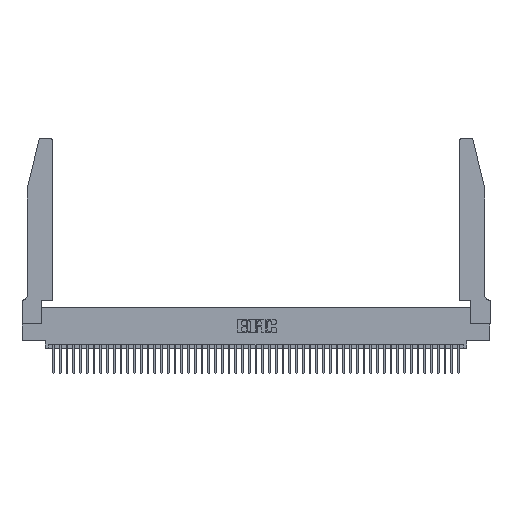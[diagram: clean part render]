
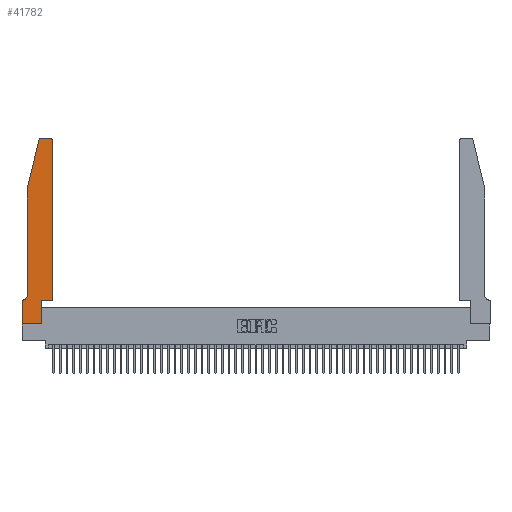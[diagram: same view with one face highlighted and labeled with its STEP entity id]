
A CAD part, top view. The second image highlights one B-rep face of the part: STEP entity #41782.
In plain terms, the highlighted planar face has unit normal (0, 0, 1).
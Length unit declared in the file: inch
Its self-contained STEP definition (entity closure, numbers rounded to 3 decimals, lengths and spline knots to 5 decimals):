
#335 = DIRECTION ( 'NONE',  ( 0., 0., 1. ) ) ;
#446 = VECTOR ( 'NONE', #50168, 39.37008 ) ;
#888 = ORIENTED_EDGE ( 'NONE', *, *, #5097, .T. ) ;
#3305 = ORIENTED_EDGE ( 'NONE', *, *, #12904, .T. ) ;
#3406 = EDGE_CURVE ( 'NONE', #11469, #32668, #41347, .T. ) ;
#3978 = VERTEX_POINT ( 'NONE', #6735 ) ;
#4355 = LINE ( 'NONE', #41577, #32899 ) ;
#4469 = DIRECTION ( 'NONE',  ( 0., 0., -1. ) ) ;
#5052 = VECTOR ( 'NONE', #42240, 39.37008 ) ;
#5097 = EDGE_CURVE ( 'NONE', #18973, #18707, #19340, .T. ) ;
#5309 = DIRECTION ( 'NONE',  ( 0., 0., 1. ) ) ;
#5389 = LINE ( 'NONE', #21109, #25408 ) ;
#5533 = EDGE_CURVE ( 'NONE', #21859, #3978, #30871, .T. ) ;
#6735 = CARTESIAN_POINT ( 'NONE',  ( 0.4205, 2.75, 0.37 ) ) ;
#6910 = EDGE_CURVE ( 'NONE', #35512, #21859, #24054, .T. ) ;
#7322 = CARTESIAN_POINT ( 'NONE',  ( 0., 0., 0.37 ) ) ;
#8686 = AXIS2_PLACEMENT_3D ( 'NONE', #47354, #4469, #46852 ) ;
#10086 = EDGE_CURVE ( 'NONE', #29222, #35360, #40199, .T. ) ;
#10791 = CARTESIAN_POINT ( 'NONE',  ( 0.284, 2.75, 0.37 ) ) ;
#11469 = VERTEX_POINT ( 'NONE', #32171 ) ;
#11515 = CARTESIAN_POINT ( 'NONE',  ( 0.4505, 0.35, 0.37 ) ) ;
#12031 = CARTESIAN_POINT ( 'NONE',  ( 0.0755, 0.42, 0.37 ) ) ;
#12190 = CARTESIAN_POINT ( 'NONE',  ( 0.4505, 0.35, 0.37 ) ) ;
#12241 = CARTESIAN_POINT ( 'NONE',  ( 0.4505, 2.72, 0.37 ) ) ;
#12771 = VERTEX_POINT ( 'NONE', #32557 ) ;
#12904 = EDGE_CURVE ( 'NONE', #12771, #30548, #36327, .T. ) ;
#13522 = ORIENTED_EDGE ( 'NONE', *, *, #5533, .T. ) ;
#13536 = LINE ( 'NONE', #14975, #5052 ) ;
#13744 = VECTOR ( 'NONE', #50152, 39.37008 ) ;
#14975 = CARTESIAN_POINT ( 'NONE',  ( 0., 0., 0.37 ) ) ;
#16902 = DIRECTION ( 'NONE',  ( -0.239, -0.971, 0. ) ) ;
#17101 = DIRECTION ( 'NONE',  ( 0., 0., 1. ) ) ;
#17632 = CARTESIAN_POINT ( 'NONE',  ( 0.0755, 0.35, 0.37 ) ) ;
#18300 = ORIENTED_EDGE ( 'NONE', *, *, #29559, .T. ) ;
#18707 = VERTEX_POINT ( 'NONE', #44211 ) ;
#18973 = VERTEX_POINT ( 'NONE', #10791 ) ;
#19340 = CIRCLE ( 'NONE', #34306, 0.03 ) ;
#19495 = EDGE_CURVE ( 'NONE', #35360, #35512, #4355, .T. ) ;
#20684 = EDGE_LOOP ( 'NONE', ( #49990, #888, #25236, #41592, #18300, #3305, #41194, #24878, #39655, #31761, #39203, #13522 ) ) ;
#20696 = CARTESIAN_POINT ( 'NONE',  ( 0., 0., 0.37 ) ) ;
#21109 = CARTESIAN_POINT ( 'NONE',  ( 0.0755, 2., 0.37 ) ) ;
#21523 = DIRECTION ( 'NONE',  ( -1., 0., 0. ) ) ;
#21859 = VERTEX_POINT ( 'NONE', #12241 ) ;
#21994 = CIRCLE ( 'NONE', #8686, 0.07 ) ;
#23254 = CARTESIAN_POINT ( 'NONE',  ( 0.284, 2.72, 0.37 ) ) ;
#24054 = LINE ( 'NONE', #12190, #13744 ) ;
#24582 = AXIS2_PLACEMENT_3D ( 'NONE', #40627, #17101, #29290 ) ;
#24878 = ORIENTED_EDGE ( 'NONE', *, *, #46065, .T. ) ;
#25236 = ORIENTED_EDGE ( 'NONE', *, *, #45693, .T. ) ;
#25249 = EDGE_CURVE ( 'NONE', #3978, #18973, #26533, .T. ) ;
#25408 = VECTOR ( 'NONE', #16902, 39.37008 ) ;
#26160 = DIRECTION ( 'NONE',  ( 1., 0., 0. ) ) ;
#26533 = LINE ( 'NONE', #34922, #446 ) ;
#26850 = VECTOR ( 'NONE', #31368, 39.37008 ) ;
#27152 = CARTESIAN_POINT ( 'NONE',  ( 0.2865, 0.35, 0.37 ) ) ;
#28473 = PLANE ( 'NONE',  #40858 ) ;
#29057 = LINE ( 'NONE', #7322, #45968 ) ;
#29222 = VERTEX_POINT ( 'NONE', #31750 ) ;
#29290 = DIRECTION ( 'NONE',  ( 1., 0., 0. ) ) ;
#29559 = EDGE_CURVE ( 'NONE', #32668, #12771, #21994, .T. ) ;
#30073 = DIRECTION ( 'NONE',  ( 1., 0., 0. ) ) ;
#30548 = VERTEX_POINT ( 'NONE', #45387 ) ;
#30871 = CIRCLE ( 'NONE', #24582, 0.03 ) ;
#31368 = DIRECTION ( 'NONE',  ( 0., 1., 0. ) ) ;
#31750 = CARTESIAN_POINT ( 'NONE',  ( 0.2865, 0., 0.37 ) ) ;
#31761 = ORIENTED_EDGE ( 'NONE', *, *, #19495, .T. ) ;
#32171 = CARTESIAN_POINT ( 'NONE',  ( 0.0755, 2., 0.37 ) ) ;
#32557 = CARTESIAN_POINT ( 'NONE',  ( 0.0055, 0.35, 0.37 ) ) ;
#32668 = VERTEX_POINT ( 'NONE', #12031 ) ;
#32899 = VECTOR ( 'NONE', #30073, 39.37008 ) ;
#33921 = VECTOR ( 'NONE', #21523, 39.37008 ) ;
#34306 = AXIS2_PLACEMENT_3D ( 'NONE', #23254, #335, #43058 ) ;
#34922 = CARTESIAN_POINT ( 'NONE',  ( 0.2605, 2.75, 0.37 ) ) ;
#35360 = VERTEX_POINT ( 'NONE', #44422 ) ;
#35512 = VERTEX_POINT ( 'NONE', #11515 ) ;
#36327 = LINE ( 'NONE', #17632, #33921 ) ;
#36858 = EDGE_CURVE ( 'NONE', #30548, #49402, #13536, .T. ) ;
#37831 = CARTESIAN_POINT ( 'NONE',  ( 0.0755, 2., 0.37 ) ) ;
#38915 = VECTOR ( 'NONE', #50025, 39.37008 ) ;
#39203 = ORIENTED_EDGE ( 'NONE', *, *, #6910, .T. ) ;
#39655 = ORIENTED_EDGE ( 'NONE', *, *, #10086, .T. ) ;
#40199 = LINE ( 'NONE', #27152, #26850 ) ;
#40627 = CARTESIAN_POINT ( 'NONE',  ( 0.4205, 2.72, 0.37 ) ) ;
#40858 = AXIS2_PLACEMENT_3D ( 'NONE', #47025, #5309, #26160 ) ;
#41194 = ORIENTED_EDGE ( 'NONE', *, *, #36858, .T. ) ;
#41347 = LINE ( 'NONE', #37831, #38915 ) ;
#41577 = CARTESIAN_POINT ( 'NONE',  ( 0.4505, 0.35, 0.37 ) ) ;
#41592 = ORIENTED_EDGE ( 'NONE', *, *, #3406, .T. ) ;
#41782 = ADVANCED_FACE ( 'NONE', ( #48294 ), #28473, .T. ) ;
#42240 = DIRECTION ( 'NONE',  ( 0., -1., 0. ) ) ;
#43058 = DIRECTION ( 'NONE',  ( 1., 0., 0. ) ) ;
#44211 = CARTESIAN_POINT ( 'NONE',  ( 0.25487, 2.72718, 0.37 ) ) ;
#44422 = CARTESIAN_POINT ( 'NONE',  ( 0.2865, 0.35, 0.37 ) ) ;
#45387 = CARTESIAN_POINT ( 'NONE',  ( 0., 0.35, 0.37 ) ) ;
#45693 = EDGE_CURVE ( 'NONE', #18707, #11469, #5389, .T. ) ;
#45968 = VECTOR ( 'NONE', #46312, 39.37008 ) ;
#46065 = EDGE_CURVE ( 'NONE', #49402, #29222, #29057, .T. ) ;
#46312 = DIRECTION ( 'NONE',  ( 1., 0., 0. ) ) ;
#46852 = DIRECTION ( 'NONE',  ( -1., 0., 0. ) ) ;
#47025 = CARTESIAN_POINT ( 'NONE',  ( 0., 0.35, 0.37 ) ) ;
#47354 = CARTESIAN_POINT ( 'NONE',  ( 0.0055, 0.42, 0.37 ) ) ;
#48294 = FACE_OUTER_BOUND ( 'NONE', #20684, .T. ) ;
#49402 = VERTEX_POINT ( 'NONE', #20696 ) ;
#49990 = ORIENTED_EDGE ( 'NONE', *, *, #25249, .T. ) ;
#50025 = DIRECTION ( 'NONE',  ( 0., -1., 0. ) ) ;
#50152 = DIRECTION ( 'NONE',  ( 0., 1., 0. ) ) ;
#50168 = DIRECTION ( 'NONE',  ( -1., 0., 0. ) ) ;
